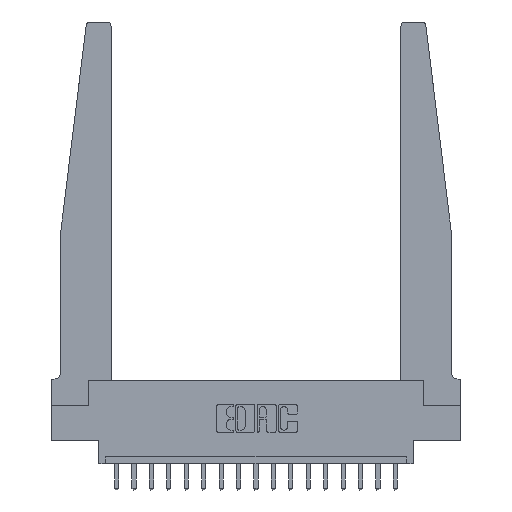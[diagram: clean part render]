
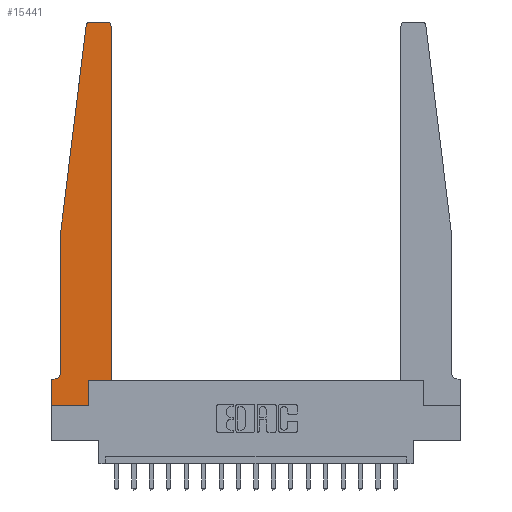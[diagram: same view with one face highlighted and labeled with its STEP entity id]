
A CAD part, top view. The second image highlights one B-rep face of the part: STEP entity #15441.
In plain terms, the highlighted planar face has unit normal (0, 0, 1).
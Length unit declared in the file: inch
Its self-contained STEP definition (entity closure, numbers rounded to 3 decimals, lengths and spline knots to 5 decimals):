
#167 = CARTESIAN_POINT ( 'NONE',  ( 0., 0.1875, 0.37 ) ) ;
#202 = EDGE_CURVE ( 'NONE', #17793, #18276, #13895, .T. ) ;
#208 = VERTEX_POINT ( 'NONE', #8472 ) ;
#293 = AXIS2_PLACEMENT_3D ( 'NONE', #13003, #14565, #7068 ) ;
#359 = VECTOR ( 'NONE', #9142, 39.37008 ) ;
#445 = CARTESIAN_POINT ( 'NONE',  ( 0., 0.1875, 0.37 ) ) ;
#739 = CARTESIAN_POINT ( 'NONE',  ( 0.065, 0.1875, 0.37 ) ) ;
#748 = VERTEX_POINT ( 'NONE', #16050 ) ;
#839 = EDGE_LOOP ( 'NONE', ( #7281, #9602, #1806, #6156, #3708, #18715, #6649, #16848, #4182, #15048, #9399, #2526 ) ) ;
#887 = VECTOR ( 'NONE', #16315, 39.37008 ) ;
#925 = EDGE_CURVE ( 'NONE', #16660, #208, #3581, .T. ) ;
#938 = CARTESIAN_POINT ( 'NONE',  ( 0.065, 0.2375, 0.37 ) ) ;
#966 = LINE ( 'NONE', #3668, #4247 ) ;
#1267 = CARTESIAN_POINT ( 'NONE',  ( 0.25, 2.75, 0.37 ) ) ;
#1438 = DIRECTION ( 'NONE',  ( 0., 0., -1. ) ) ;
#1662 = CARTESIAN_POINT ( 'NONE',  ( 0.425, 0.18, 0.37 ) ) ;
#1806 = ORIENTED_EDGE ( 'NONE', *, *, #1949, .T. ) ;
#1949 = EDGE_CURVE ( 'NONE', #5992, #4051, #966, .T. ) ;
#2173 = DIRECTION ( 'NONE',  ( -1., 0., 0. ) ) ;
#2195 = DIRECTION ( 'NONE',  ( 1., 0., 0. ) ) ;
#2526 = ORIENTED_EDGE ( 'NONE', *, *, #14446, .T. ) ;
#3139 = PLANE ( 'NONE',  #17022 ) ;
#3266 = VECTOR ( 'NONE', #5607, 39.37008 ) ;
#3581 = LINE ( 'NONE', #4777, #359 ) ;
#3583 = DIRECTION ( 'NONE',  ( 0., 0., 1. ) ) ;
#3668 = CARTESIAN_POINT ( 'NONE',  ( 0.065, 1.25, 0.37 ) ) ;
#3708 = ORIENTED_EDGE ( 'NONE', *, *, #4066, .T. ) ;
#4051 = VERTEX_POINT ( 'NONE', #18059 ) ;
#4066 = EDGE_CURVE ( 'NONE', #17407, #11701, #11676, .T. ) ;
#4128 = VERTEX_POINT ( 'NONE', #167 ) ;
#4182 = ORIENTED_EDGE ( 'NONE', *, *, #202, .T. ) ;
#4226 = CARTESIAN_POINT ( 'NONE',  ( 0.395, 2.75, 0.37 ) ) ;
#4247 = VECTOR ( 'NONE', #5282, 39.37008 ) ;
#4681 = DIRECTION ( 'NONE',  ( 0., 0., 1. ) ) ;
#4712 = CARTESIAN_POINT ( 'NONE',  ( 0.015, 0.2375, 0.37 ) ) ;
#4743 = CARTESIAN_POINT ( 'NONE',  ( 0.2605, 0., 0.37 ) ) ;
#4777 = CARTESIAN_POINT ( 'NONE',  ( 0.425, 0.18, 0.37 ) ) ;
#4972 = EDGE_CURVE ( 'NONE', #4128, #16677, #18018, .T. ) ;
#5217 = LINE ( 'NONE', #739, #17054 ) ;
#5282 = DIRECTION ( 'NONE',  ( -0.122, -0.992, 0. ) ) ;
#5607 = DIRECTION ( 'NONE',  ( -1., 0., 0. ) ) ;
#5714 = DIRECTION ( 'NONE',  ( 0., -1., 0. ) ) ;
#5732 = CARTESIAN_POINT ( 'NONE',  ( 0.425, 0.18, 0.37 ) ) ;
#5776 = CARTESIAN_POINT ( 'NONE',  ( 0.2605, 0.18, 0.37 ) ) ;
#5849 = LINE ( 'NONE', #11621, #15184 ) ;
#5853 = CARTESIAN_POINT ( 'NONE',  ( 0.2605, 0.18, 0.37 ) ) ;
#5992 = VERTEX_POINT ( 'NONE', #7252 ) ;
#6156 = ORIENTED_EDGE ( 'NONE', *, *, #18115, .T. ) ;
#6433 = AXIS2_PLACEMENT_3D ( 'NONE', #16659, #3583, #2195 ) ;
#6506 = AXIS2_PLACEMENT_3D ( 'NONE', #4712, #1438, #13356 ) ;
#6511 = CIRCLE ( 'NONE', #293, 0.03 ) ;
#6649 = ORIENTED_EDGE ( 'NONE', *, *, #4972, .T. ) ;
#7068 = DIRECTION ( 'NONE',  ( 1., 0., 0. ) ) ;
#7142 = LINE ( 'NONE', #1267, #3266 ) ;
#7252 = CARTESIAN_POINT ( 'NONE',  ( 0.24675, 2.72367, 0.37 ) ) ;
#7281 = ORIENTED_EDGE ( 'NONE', *, *, #12719, .T. ) ;
#7297 = EDGE_CURVE ( 'NONE', #11701, #4128, #5217, .T. ) ;
#8472 = CARTESIAN_POINT ( 'NONE',  ( 0.425, 2.72, 0.37 ) ) ;
#8703 = VERTEX_POINT ( 'NONE', #4226 ) ;
#8709 = LINE ( 'NONE', #14107, #9445 ) ;
#9142 = DIRECTION ( 'NONE',  ( 0., 1., 0. ) ) ;
#9399 = ORIENTED_EDGE ( 'NONE', *, *, #925, .T. ) ;
#9445 = VECTOR ( 'NONE', #17211, 39.37008 ) ;
#9602 = ORIENTED_EDGE ( 'NONE', *, *, #18719, .T. ) ;
#9620 = LINE ( 'NONE', #1662, #887 ) ;
#11091 = CARTESIAN_POINT ( 'NONE',  ( 0.015, 0.1875, 0.37 ) ) ;
#11140 = VECTOR ( 'NONE', #13284, 39.37008 ) ;
#11208 = CIRCLE ( 'NONE', #6433, 0.03 ) ;
#11621 = CARTESIAN_POINT ( 'NONE',  ( 0.065, 1.25, 0.37 ) ) ;
#11676 = CIRCLE ( 'NONE', #6506, 0.05 ) ;
#11701 = VERTEX_POINT ( 'NONE', #11091 ) ;
#12634 = DIRECTION ( 'NONE',  ( 0., -1., 0. ) ) ;
#12719 = EDGE_CURVE ( 'NONE', #8703, #748, #7142, .T. ) ;
#12970 = CARTESIAN_POINT ( 'NONE',  ( 0., 0., 0.37 ) ) ;
#13003 = CARTESIAN_POINT ( 'NONE',  ( 0.27653, 2.72, 0.37 ) ) ;
#13094 = EDGE_CURVE ( 'NONE', #16677, #17793, #8709, .T. ) ;
#13284 = DIRECTION ( 'NONE',  ( 0., 1., 0. ) ) ;
#13356 = DIRECTION ( 'NONE',  ( -1., 0., 0. ) ) ;
#13895 = LINE ( 'NONE', #5776, #11140 ) ;
#14019 = EDGE_CURVE ( 'NONE', #18276, #16660, #9620, .T. ) ;
#14107 = CARTESIAN_POINT ( 'NONE',  ( 0., 0., 0.37 ) ) ;
#14446 = EDGE_CURVE ( 'NONE', #208, #8703, #11208, .T. ) ;
#14565 = DIRECTION ( 'NONE',  ( 0., 0., 1. ) ) ;
#14861 = DIRECTION ( 'NONE',  ( 1., 0., 0. ) ) ;
#15048 = ORIENTED_EDGE ( 'NONE', *, *, #14019, .T. ) ;
#15184 = VECTOR ( 'NONE', #5714, 39.37008 ) ;
#15441 = ADVANCED_FACE ( 'NONE', ( #17517 ), #3139, .T. ) ;
#16050 = CARTESIAN_POINT ( 'NONE',  ( 0.27653, 2.75, 0.37 ) ) ;
#16315 = DIRECTION ( 'NONE',  ( 1., 0., 0. ) ) ;
#16659 = CARTESIAN_POINT ( 'NONE',  ( 0.395, 2.72, 0.37 ) ) ;
#16660 = VERTEX_POINT ( 'NONE', #5732 ) ;
#16677 = VERTEX_POINT ( 'NONE', #12970 ) ;
#16848 = ORIENTED_EDGE ( 'NONE', *, *, #13094, .T. ) ;
#17022 = AXIS2_PLACEMENT_3D ( 'NONE', #445, #4681, #14861 ) ;
#17054 = VECTOR ( 'NONE', #2173, 39.37008 ) ;
#17211 = DIRECTION ( 'NONE',  ( 1., 0., 0. ) ) ;
#17407 = VERTEX_POINT ( 'NONE', #938 ) ;
#17517 = FACE_OUTER_BOUND ( 'NONE', #839, .T. ) ;
#17793 = VERTEX_POINT ( 'NONE', #4743 ) ;
#18018 = LINE ( 'NONE', #18530, #18673 ) ;
#18059 = CARTESIAN_POINT ( 'NONE',  ( 0.065, 1.25, 0.37 ) ) ;
#18115 = EDGE_CURVE ( 'NONE', #4051, #17407, #5849, .T. ) ;
#18276 = VERTEX_POINT ( 'NONE', #5853 ) ;
#18530 = CARTESIAN_POINT ( 'NONE',  ( 0., 0., 0.37 ) ) ;
#18673 = VECTOR ( 'NONE', #12634, 39.37008 ) ;
#18715 = ORIENTED_EDGE ( 'NONE', *, *, #7297, .T. ) ;
#18719 = EDGE_CURVE ( 'NONE', #748, #5992, #6511, .T. ) ;
